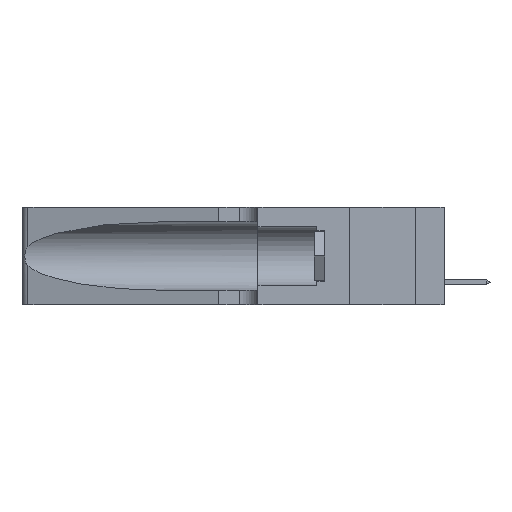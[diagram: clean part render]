
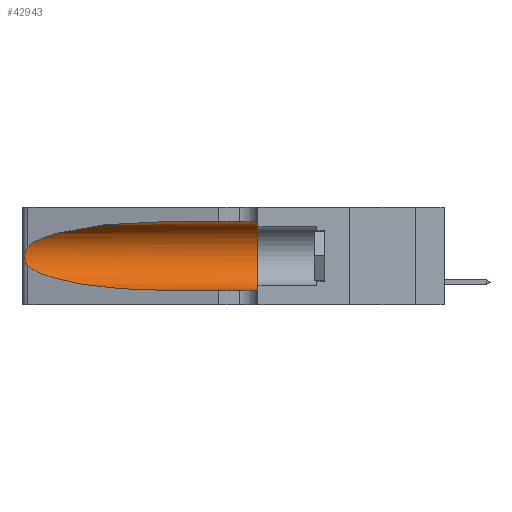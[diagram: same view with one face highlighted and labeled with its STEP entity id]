
A CAD part, left-side view. The second image highlights one B-rep face of the part: STEP entity #42943.
In plain terms, the highlighted cylindrical face has radius 3.308 mm (diameter 6.617 mm), a partial arc.
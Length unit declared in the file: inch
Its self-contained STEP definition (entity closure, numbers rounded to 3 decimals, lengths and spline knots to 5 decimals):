
#361 = ORIENTED_EDGE ( 'NONE', *, *, #4116, .T. ) ;
#665 = CARTESIAN_POINT ( 'NONE',  ( 0.25487, 1.22718, 0.22369 ) ) ;
#1196 = ORIENTED_EDGE ( 'NONE', *, *, #36170, .F. ) ;
#2134 = VECTOR ( 'NONE', #48744, 39.37008 ) ;
#2464 = VERTEX_POINT ( 'NONE', #49739 ) ;
#2870 = CARTESIAN_POINT ( 'NONE',  ( 0.26017, 1.23833, 0.17102 ) ) ;
#3061 = CARTESIAN_POINT ( 'NONE',  ( 0.25555, 1.22994, 0.2215 ) ) ;
#3245 = CARTESIAN_POINT ( 'NONE',  ( 0.25555, 1.22993, 0.14849 ) ) ;
#3627 = CARTESIAN_POINT ( 'NONE',  ( 0.2373, 1.15595, 0.28018 ) ) ;
#4116 = EDGE_CURVE ( 'NONE', #42720, #37817, #41867, .T. ) ;
#5512 = CARTESIAN_POINT ( 'NONE',  ( 0.18966, 0.96281, 0.05475 ) ) ;
#5597 = VERTEX_POINT ( 'NONE', #42727 ) ;
#5694 = B_SPLINE_CURVE_WITH_KNOTS ( 'NONE', 3,
 ( #26491, #3061, #7356, #38630, #42564, #27005, #50460, #50114, #2870, #34691, #7023, #19112, #3245, #34526 ),
 .UNSPECIFIED., .F., .F.,
 ( 4, 2, 2, 2, 2, 2, 4 ),
 ( 0., 0.00027, 0.00053, 0.00107, 0.0016, 0.00187, 0.00214 ),
 .UNSPECIFIED. ) ;
#7023 = CARTESIAN_POINT ( 'NONE',  ( 0.25789, 1.23486, 0.15765 ) ) ;
#7356 = CARTESIAN_POINT ( 'NONE',  ( 0.25639, 1.23184, 0.21858 ) ) ;
#11804 = FACE_OUTER_BOUND ( 'NONE', #39126, .T. ) ;
#11934 = CARTESIAN_POINT ( 'NONE',  ( 0.1305, 0.72297, 0.05475 ) ) ;
#13531 = ORIENTED_EDGE ( 'NONE', *, *, #19217, .F. ) ;
#14260 = CARTESIAN_POINT ( 'NONE',  ( 0.1305, 1.61858, 0.185 ) ) ;
#14314 = EDGE_CURVE ( 'NONE', #37817, #31481, #17309, .T. ) ;
#16622 = EDGE_CURVE ( 'NONE', #5597, #42720, #5694, .T. ) ;
#16778 = CARTESIAN_POINT ( 'NONE',  ( 0.1305, 0.72297, 0.05475 ) ) ;
#17309 = LINE ( 'NONE', #41426, #22295 ) ;
#17982 = DIRECTION ( 'NONE',  ( 0., -1., 0. ) ) ;
#19112 = CARTESIAN_POINT ( 'NONE',  ( 0.25639, 1.23186, 0.15144 ) ) ;
#19217 = EDGE_CURVE ( 'NONE', #2464, #31481, #36524, .T. ) ;
#20268 = CARTESIAN_POINT ( 'NONE',  ( 0.1305, 0.35, 0.185 ) ) ;
#22096 = CARTESIAN_POINT ( 'NONE',  ( 0.1305, 0.35, 0.05475 ) ) ;
#22295 = VECTOR ( 'NONE', #17982, 39.37008 ) ;
#22658 = ORIENTED_EDGE ( 'NONE', *, *, #16622, .T. ) ;
#22812 = DIRECTION ( 'NONE',  ( 0., 1., 0. ) ) ;
#23775 = DIRECTION ( 'NONE',  ( 0., 0., 1. ) ) ;
#24161 = LINE ( 'NONE', #44300, #2134 ) ;
#24829 = CARTESIAN_POINT ( 'NONE',  ( 0.2373, 1.15595, 0.08982 ) ) ;
#26491 = CARTESIAN_POINT ( 'NONE',  ( 0.25487, 1.22718, 0.22369 ) ) ;
#26492 = CYLINDRICAL_SURFACE ( 'NONE', #44469, 0.13025 ) ;
#26579 = DIRECTION ( 'NONE',  ( 0., -1., 0. ) ) ;
#27005 = CARTESIAN_POINT ( 'NONE',  ( 0.26018, 1.23835, 0.19895 ) ) ;
#27379 = CARTESIAN_POINT ( 'NONE',  ( 0.1305, 0.72297, 0.31525 ) ) ;
#31481 = VERTEX_POINT ( 'NONE', #22096 ) ;
#33595 = EDGE_CURVE ( 'NONE', #44232, #5597, #45280, .T. ) ;
#34446 = DIRECTION ( 'NONE',  ( 0., 0., -1. ) ) ;
#34526 = CARTESIAN_POINT ( 'NONE',  ( 0.25487, 1.22718, 0.14631 ) ) ;
#34691 = CARTESIAN_POINT ( 'NONE',  ( 0.25856, 1.23593, 0.16098 ) ) ;
#36170 = EDGE_CURVE ( 'NONE', #44232, #2464, #24161, .T. ) ;
#36524 = CIRCLE ( 'NONE', #46709, 0.13025 ) ;
#37817 = VERTEX_POINT ( 'NONE', #11934 ) ;
#38374 = ORIENTED_EDGE ( 'NONE', *, *, #33595, .T. ) ;
#38630 = CARTESIAN_POINT ( 'NONE',  ( 0.25787, 1.23484, 0.2124 ) ) ;
#39126 = EDGE_LOOP ( 'NONE', ( #38374, #22658, #361, #44775, #13531, #1196 ) ) ;
#41426 = CARTESIAN_POINT ( 'NONE',  ( 0.1305, 1.61858, 0.05475 ) ) ;
#41459 = CARTESIAN_POINT ( 'NONE',  ( 0.1305, 0.72297, 0.31525 ) ) ;
#41867 =( BOUNDED_CURVE ( )  B_SPLINE_CURVE ( 3, ( #44892, #24829, #5512, #16778 ),
 .UNSPECIFIED., .F., .T. ) 
 B_SPLINE_CURVE_WITH_KNOTS ( ( 4, 4 ),
 ( 3.44316, 4.71239 ),
 .UNSPECIFIED. ) 
 CURVE ( )  GEOMETRIC_REPRESENTATION_ITEM ( )  RATIONAL_B_SPLINE_CURVE ( ( 1., 0.87, 0.87, 1. ) ) 
 REPRESENTATION_ITEM ( '' )  );
#42564 = CARTESIAN_POINT ( 'NONE',  ( 0.25854, 1.2359, 0.20912 ) ) ;
#42720 = VERTEX_POINT ( 'NONE', #44477 ) ;
#42727 = CARTESIAN_POINT ( 'NONE',  ( 0.25487, 1.22718, 0.22369 ) ) ;
#42943 = ADVANCED_FACE ( 'NONE', ( #11804 ), #26492, .F. ) ;
#44232 = VERTEX_POINT ( 'NONE', #41459 ) ;
#44300 = CARTESIAN_POINT ( 'NONE',  ( 0.1305, 1.61858, 0.31525 ) ) ;
#44469 = AXIS2_PLACEMENT_3D ( 'NONE', #14260, #26579, #34446 ) ;
#44477 = CARTESIAN_POINT ( 'NONE',  ( 0.25487, 1.22718, 0.14631 ) ) ;
#44775 = ORIENTED_EDGE ( 'NONE', *, *, #14314, .T. ) ;
#44892 = CARTESIAN_POINT ( 'NONE',  ( 0.25487, 1.22718, 0.14631 ) ) ;
#45280 =( BOUNDED_CURVE ( )  B_SPLINE_CURVE ( 3, ( #27379, #46421, #3627, #665 ),
 .UNSPECIFIED., .F., .T. ) 
 B_SPLINE_CURVE_WITH_KNOTS ( ( 4, 4 ),
 ( 1.5708, 2.84003 ),
 .UNSPECIFIED. ) 
 CURVE ( )  GEOMETRIC_REPRESENTATION_ITEM ( )  RATIONAL_B_SPLINE_CURVE ( ( 1., 0.87, 0.87, 1. ) ) 
 REPRESENTATION_ITEM ( '' )  );
#46421 = CARTESIAN_POINT ( 'NONE',  ( 0.18966, 0.96281, 0.31525 ) ) ;
#46709 = AXIS2_PLACEMENT_3D ( 'NONE', #20268, #22812, #23775 ) ;
#48744 = DIRECTION ( 'NONE',  ( 0., -1., 0. ) ) ;
#49739 = CARTESIAN_POINT ( 'NONE',  ( 0.1305, 0.35, 0.31525 ) ) ;
#50114 = CARTESIAN_POINT ( 'NONE',  ( 0.26075, 1.23896, 0.178 ) ) ;
#50460 = CARTESIAN_POINT ( 'NONE',  ( 0.26075, 1.23896, 0.19203 ) ) ;
